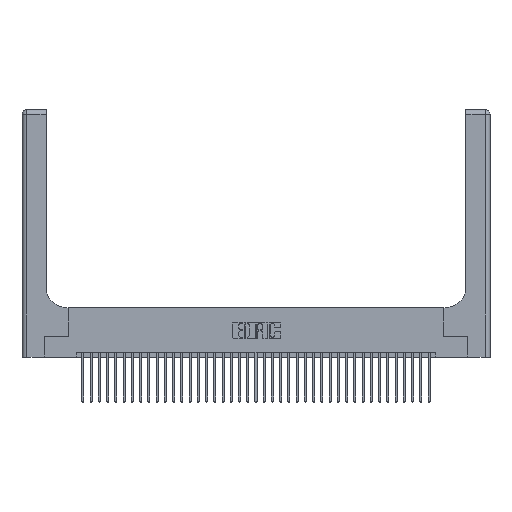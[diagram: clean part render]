
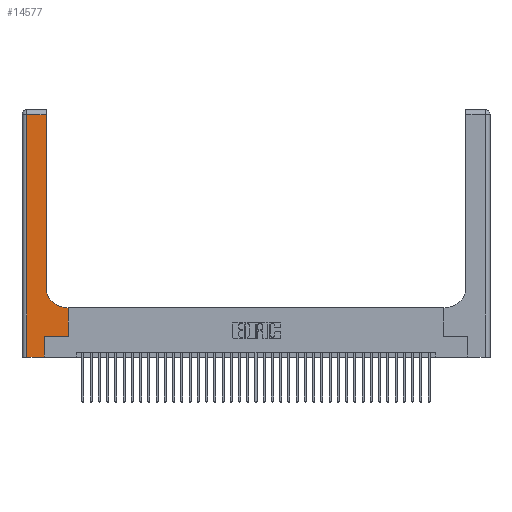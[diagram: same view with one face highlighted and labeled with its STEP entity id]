
A CAD part, top view. The second image highlights one B-rep face of the part: STEP entity #14577.
In plain terms, the highlighted planar face has unit normal (0, 0, 1).
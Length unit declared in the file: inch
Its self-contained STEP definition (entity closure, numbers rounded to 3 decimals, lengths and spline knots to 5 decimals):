
#78 = CARTESIAN_POINT ( 'NONE',  ( 0.269, 0., 0.37 ) ) ;
#135 = CARTESIAN_POINT ( 'NONE',  ( 0.269, 0., 0.37 ) ) ;
#1649 = CARTESIAN_POINT ( 'NONE',  ( 0., 0., 0.37 ) ) ;
#3159 = ORIENTED_EDGE ( 'NONE', *, *, #4408, .T. ) ;
#3562 = LINE ( 'NONE', #11890, #20342 ) ;
#3612 = ORIENTED_EDGE ( 'NONE', *, *, #13307, .T. ) ;
#4240 = ORIENTED_EDGE ( 'NONE', *, *, #22685, .T. ) ;
#4408 = EDGE_CURVE ( 'NONE', #6453, #7287, #33554, .T. ) ;
#6453 = VERTEX_POINT ( 'NONE', #24191 ) ;
#7287 = VERTEX_POINT ( 'NONE', #15484 ) ;
#8035 = CARTESIAN_POINT ( 'NONE',  ( 0.2915, 2.94, 0.37 ) ) ;
#8629 = VERTEX_POINT ( 'NONE', #20333 ) ;
#8644 = EDGE_CURVE ( 'NONE', #38144, #35610, #3562, .T. ) ;
#9552 = VECTOR ( 'NONE', #22380, 39.37008 ) ;
#9782 = ORIENTED_EDGE ( 'NONE', *, *, #28694, .T. ) ;
#10185 = CARTESIAN_POINT ( 'NONE',  ( 0.5585, 0.6, 0.37 ) ) ;
#10541 = ORIENTED_EDGE ( 'NONE', *, *, #8644, .T. ) ;
#11086 = DIRECTION ( 'NONE',  ( -1., 0., 0. ) ) ;
#11705 = LINE ( 'NONE', #35854, #17266 ) ;
#11890 = CARTESIAN_POINT ( 'NONE',  ( 0.269, 0.25, 0.37 ) ) ;
#12070 = CARTESIAN_POINT ( 'NONE',  ( 0.5415, 0.85, 0.37 ) ) ;
#13307 = EDGE_CURVE ( 'NONE', #7287, #35569, #20583, .T. ) ;
#14577 = ADVANCED_FACE ( 'NONE', ( #20508 ), #34408, .F. ) ;
#15139 = VECTOR ( 'NONE', #11086, 39.37008 ) ;
#15484 = CARTESIAN_POINT ( 'NONE',  ( 0.06, 0., 0.37 ) ) ;
#16180 = CARTESIAN_POINT ( 'NONE',  ( 0.5585, 0.25, 0.37 ) ) ;
#16202 = CARTESIAN_POINT ( 'NONE',  ( 0.269, 0.25, 0.37 ) ) ;
#17266 = VECTOR ( 'NONE', #20918, 39.37008 ) ;
#17342 = DIRECTION ( 'NONE',  ( 1., 0., 0. ) ) ;
#17657 = DIRECTION ( 'NONE',  ( 0., 0., -1. ) ) ;
#18187 = DIRECTION ( 'NONE',  ( 0., 1., 0. ) ) ;
#18193 = ORIENTED_EDGE ( 'NONE', *, *, #34827, .T. ) ;
#19419 = DIRECTION ( 'NONE',  ( -1., 0., 0. ) ) ;
#19467 = DIRECTION ( 'NONE',  ( 0., 0., -1. ) ) ;
#19527 = CARTESIAN_POINT ( 'NONE',  ( 0.2915, 0.6, 0.37 ) ) ;
#20333 = CARTESIAN_POINT ( 'NONE',  ( 0.5415, 0.6, 0.37 ) ) ;
#20342 = VECTOR ( 'NONE', #17342, 39.37008 ) ;
#20508 = FACE_OUTER_BOUND ( 'NONE', #25936, .T. ) ;
#20583 = LINE ( 'NONE', #1649, #34197 ) ;
#20909 = DIRECTION ( 'NONE',  ( 1., 0., 0. ) ) ;
#20918 = DIRECTION ( 'NONE',  ( 0., 1., 0. ) ) ;
#21917 = VECTOR ( 'NONE', #19419, 39.37008 ) ;
#22001 = VERTEX_POINT ( 'NONE', #8035 ) ;
#22249 = CIRCLE ( 'NONE', #23559, 0.25 ) ;
#22380 = DIRECTION ( 'NONE',  ( 0., 1., 0. ) ) ;
#22454 = CARTESIAN_POINT ( 'NONE',  ( 0., 3., 0.37 ) ) ;
#22685 = EDGE_CURVE ( 'NONE', #35610, #30141, #35315, .T. ) ;
#23462 = ORIENTED_EDGE ( 'NONE', *, *, #36623, .T. ) ;
#23559 = AXIS2_PLACEMENT_3D ( 'NONE', #12070, #17657, #20909 ) ;
#24191 = CARTESIAN_POINT ( 'NONE',  ( 0.06, 2.94, 0.37 ) ) ;
#24722 = EDGE_CURVE ( 'NONE', #30141, #8629, #33850, .T. ) ;
#25113 = DIRECTION ( 'NONE',  ( 1., 0., 0. ) ) ;
#25266 = DIRECTION ( 'NONE',  ( 0., -1., 0. ) ) ;
#25496 = LINE ( 'NONE', #135, #34948 ) ;
#25936 = EDGE_LOOP ( 'NONE', ( #18193, #28209, #3159, #3612, #9782, #10541, #4240, #38271, #23462 ) ) ;
#27058 = EDGE_CURVE ( 'NONE', #22001, #6453, #29880, .T. ) ;
#28209 = ORIENTED_EDGE ( 'NONE', *, *, #27058, .T. ) ;
#28694 = EDGE_CURVE ( 'NONE', #35569, #38144, #25496, .T. ) ;
#29880 = LINE ( 'NONE', #37135, #21917 ) ;
#30141 = VERTEX_POINT ( 'NONE', #10185 ) ;
#32560 = VERTEX_POINT ( 'NONE', #34234 ) ;
#32606 = VECTOR ( 'NONE', #25266, 39.37008 ) ;
#33554 = LINE ( 'NONE', #34624, #32606 ) ;
#33709 = CARTESIAN_POINT ( 'NONE',  ( 0.5585, 0.25, 0.37 ) ) ;
#33850 = LINE ( 'NONE', #19527, #15139 ) ;
#34037 = DIRECTION ( 'NONE',  ( -1., 0., 0. ) ) ;
#34197 = VECTOR ( 'NONE', #25113, 39.37008 ) ;
#34234 = CARTESIAN_POINT ( 'NONE',  ( 0.2915, 0.85, 0.37 ) ) ;
#34408 = PLANE ( 'NONE',  #37282 ) ;
#34624 = CARTESIAN_POINT ( 'NONE',  ( 0.06, 3., 0.37 ) ) ;
#34827 = EDGE_CURVE ( 'NONE', #32560, #22001, #11705, .T. ) ;
#34948 = VECTOR ( 'NONE', #18187, 39.37008 ) ;
#35315 = LINE ( 'NONE', #16180, #9552 ) ;
#35569 = VERTEX_POINT ( 'NONE', #78 ) ;
#35610 = VERTEX_POINT ( 'NONE', #33709 ) ;
#35854 = CARTESIAN_POINT ( 'NONE',  ( 0.2915, 3., 0.37 ) ) ;
#36623 = EDGE_CURVE ( 'NONE', #8629, #32560, #22249, .T. ) ;
#37135 = CARTESIAN_POINT ( 'NONE',  ( 0., 2.94, 0.37 ) ) ;
#37282 = AXIS2_PLACEMENT_3D ( 'NONE', #22454, #19467, #34037 ) ;
#38144 = VERTEX_POINT ( 'NONE', #16202 ) ;
#38271 = ORIENTED_EDGE ( 'NONE', *, *, #24722, .T. ) ;
